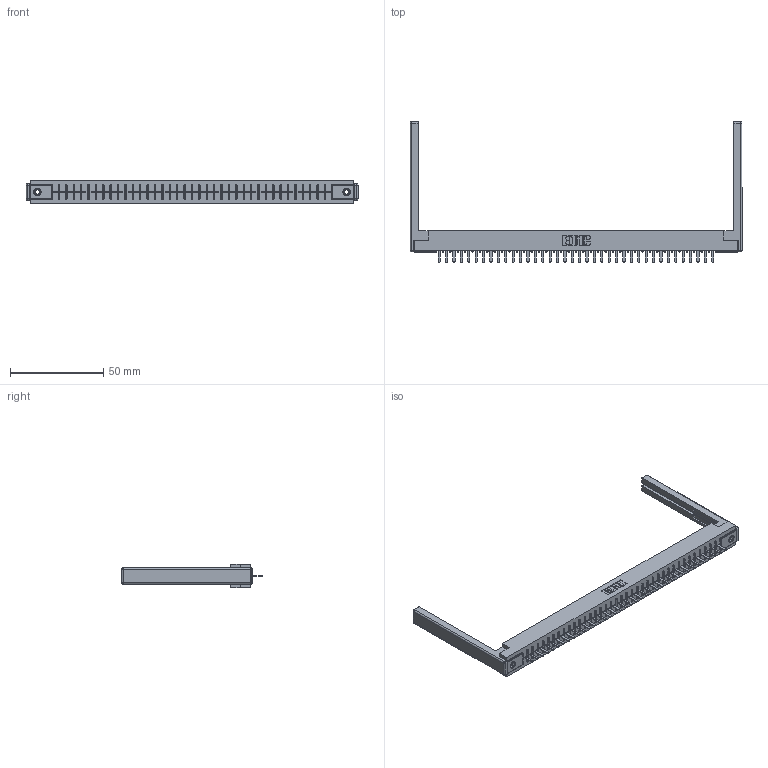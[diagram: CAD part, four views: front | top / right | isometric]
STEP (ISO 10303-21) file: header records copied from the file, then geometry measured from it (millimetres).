
FILE_DESCRIPTION (( 'STEP AP203' ), '1' );
FILE_NAME ('316-038-520-168.STEP', '2018-07-31T04:56:17', ( '' ), ( '' ), 'SwSTEP 2.0', 'SolidWorks 2016', '' );
FILE_SCHEMA (( 'CONFIG_CONTROL_DESIGN' ));
Length unit declared in the file: inch
Products named in the file (5): 306 Part_.156 Dia; 306-290-001_120; 345-250-001_345-250-001-102; 307-220-068; 316-038-520-168
Assembly tree (43 placements, depth 2):
  316-038-520-168
    306 Part_.156 Dia
    306-290-001_120  x38
    345-250-001_345-250-001-102  x2
    307-220-068  x2
Bounding box: 178 x 75.41 x 12.7 mm (x, y, z)
Volume: 24023.2 mm3; surface area: 24200.7 mm2
Topology: 43 solids, 43 shells, 2930 faces, 8192 edges, 5236 vertices
Faces by surface type: plane 1942, cylinder 812, sphere 160, cone 12, torus 4
Entity records: 38670 total; most frequent: CARTESIAN_POINT 6458, ORIENTED_EDGE 6394, DIRECTION 6381, EDGE_CURVE 3197, VECTOR 2495, LINE 2495, VERTEX_POINT 2020, AXIS2_PLACEMENT_3D 1943
